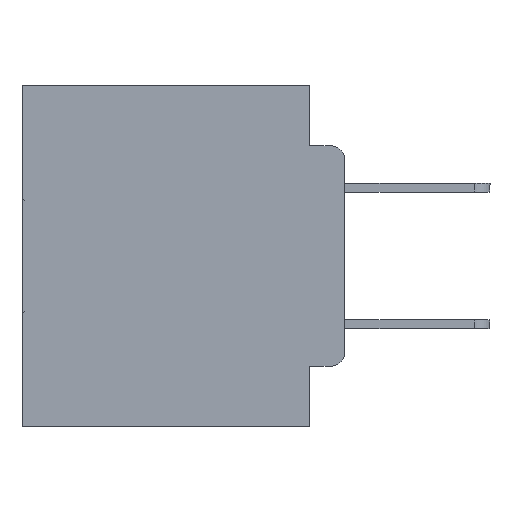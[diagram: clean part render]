
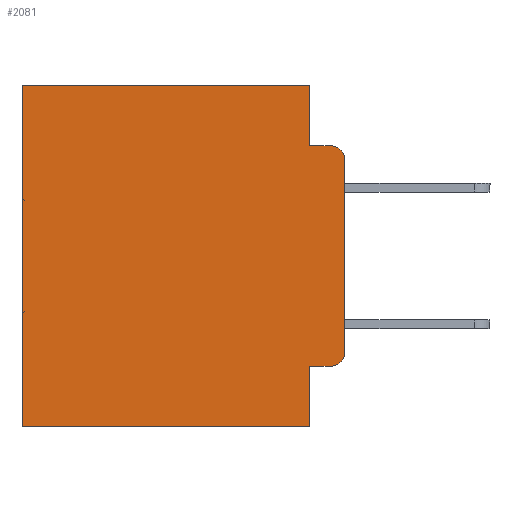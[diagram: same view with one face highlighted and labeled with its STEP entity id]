
A CAD part, left-side view. The second image highlights one B-rep face of the part: STEP entity #2081.
In plain terms, the highlighted planar face has unit normal (-1, 0, 0).
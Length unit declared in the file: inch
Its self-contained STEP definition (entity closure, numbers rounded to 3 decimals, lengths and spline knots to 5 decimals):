
#82 = CARTESIAN_POINT ( 'NONE',  ( 0.298, 0.473, -0.5 ) ) ;
#234 = CARTESIAN_POINT ( 'NONE',  ( 0.298, 0.473, 0. ) ) ;
#344 = ORIENTED_EDGE ( 'NONE', *, *, #11856, .F. ) ;
#406 = VECTOR ( 'NONE', #6582, 39.37008 ) ;
#436 = LINE ( 'NONE', #24185, #19536 ) ;
#500 = VECTOR ( 'NONE', #5711, 39.37008 ) ;
#1049 = ORIENTED_EDGE ( 'NONE', *, *, #2192, .F. ) ;
#1088 = LINE ( 'NONE', #22377, #31598 ) ;
#1251 = DIRECTION ( 'NONE',  ( -1., 0., 0. ) ) ;
#1315 = LINE ( 'NONE', #20563, #500 ) ;
#1453 = EDGE_LOOP ( 'NONE', ( #344, #12089, #8398, #3783, #7740, #3040, #1049, #2171, #7056, #9646 ) ) ;
#1758 = EDGE_CURVE ( 'NONE', #31457, #2071, #436, .T. ) ;
#2012 = CARTESIAN_POINT ( 'NONE',  ( 0.298, 0.051, -0.5 ) ) ;
#2071 = VERTEX_POINT ( 'NONE', #4036 ) ;
#2081 = ADVANCED_FACE ( 'NONE', ( #30602 ), #30395, .F. ) ;
#2091 = DIRECTION ( 'NONE',  ( 0., -1., 0. ) ) ;
#2171 = ORIENTED_EDGE ( 'NONE', *, *, #20713, .F. ) ;
#2192 = EDGE_CURVE ( 'NONE', #28449, #8129, #26793, .T. ) ;
#2549 = CARTESIAN_POINT ( 'NONE',  ( 0.298, 0.051, -0.4115 ) ) ;
#2561 = CARTESIAN_POINT ( 'NONE',  ( 0.298, 0.051, 0. ) ) ;
#3040 = ORIENTED_EDGE ( 'NONE', *, *, #22358, .T. ) ;
#3138 = CARTESIAN_POINT ( 'NONE',  ( 0.298, 0., -0.1085 ) ) ;
#3783 = ORIENTED_EDGE ( 'NONE', *, *, #27270, .F. ) ;
#4036 = CARTESIAN_POINT ( 'NONE',  ( 0.298, 0.02, -0.0885 ) ) ;
#4209 = VERTEX_POINT ( 'NONE', #234 ) ;
#5115 = DIRECTION ( 'NONE',  ( 0., 0., -1. ) ) ;
#5131 = EDGE_CURVE ( 'NONE', #28104, #2071, #10438, .T. ) ;
#5205 = VERTEX_POINT ( 'NONE', #13309 ) ;
#5264 = CARTESIAN_POINT ( 'NONE',  ( 0.298, 0.473, 0. ) ) ;
#5711 = DIRECTION ( 'NONE',  ( 0., 1., 0. ) ) ;
#6582 = DIRECTION ( 'NONE',  ( 0., 1., 0. ) ) ;
#7056 = ORIENTED_EDGE ( 'NONE', *, *, #12464, .T. ) ;
#7740 = ORIENTED_EDGE ( 'NONE', *, *, #15792, .T. ) ;
#8129 = VERTEX_POINT ( 'NONE', #82 ) ;
#8398 = ORIENTED_EDGE ( 'NONE', *, *, #1758, .F. ) ;
#8658 = LINE ( 'NONE', #2549, #21014 ) ;
#9132 = EDGE_CURVE ( 'NONE', #31596, #11874, #24035, .T. ) ;
#9646 = ORIENTED_EDGE ( 'NONE', *, *, #9132, .T. ) ;
#10153 = DIRECTION ( 'NONE',  ( 0., 0., -1. ) ) ;
#10220 = CARTESIAN_POINT ( 'NONE',  ( 0.298, 0.02, -0.1085 ) ) ;
#10438 = CIRCLE ( 'NONE', #16133, 0.02 ) ;
#11856 = EDGE_CURVE ( 'NONE', #28104, #11874, #26385, .T. ) ;
#11874 = VERTEX_POINT ( 'NONE', #29782 ) ;
#12089 = ORIENTED_EDGE ( 'NONE', *, *, #5131, .T. ) ;
#12464 = EDGE_CURVE ( 'NONE', #5205, #31596, #8658, .T. ) ;
#12546 = CARTESIAN_POINT ( 'NONE',  ( 0.298, 0.02, -0.4115 ) ) ;
#13309 = CARTESIAN_POINT ( 'NONE',  ( 0.298, 0.051, -0.4115 ) ) ;
#14399 = CARTESIAN_POINT ( 'NONE',  ( 0.298, 0.02, -0.3915 ) ) ;
#14442 = LINE ( 'NONE', #5264, #21781 ) ;
#15792 = EDGE_CURVE ( 'NONE', #24502, #4209, #1315, .T. ) ;
#16133 = AXIS2_PLACEMENT_3D ( 'NONE', #10220, #1251, #10153 ) ;
#16844 = DIRECTION ( 'NONE',  ( 0., 0., -1. ) ) ;
#17233 = VECTOR ( 'NONE', #27936, 39.37008 ) ;
#17857 = AXIS2_PLACEMENT_3D ( 'NONE', #14399, #31499, #16844 ) ;
#17874 = CARTESIAN_POINT ( 'NONE',  ( 0.298, 0., -0.5 ) ) ;
#18517 = AXIS2_PLACEMENT_3D ( 'NONE', #22506, #21951, #21909 ) ;
#19536 = VECTOR ( 'NONE', #2091, 39.37008 ) ;
#19902 = DIRECTION ( 'NONE',  ( 0., 0., -1. ) ) ;
#19928 = DIRECTION ( 'NONE',  ( 0., -1., 0. ) ) ;
#20445 = CARTESIAN_POINT ( 'NONE',  ( 0.298, 0.051, 0. ) ) ;
#20563 = CARTESIAN_POINT ( 'NONE',  ( 0.298, 0., 0. ) ) ;
#20683 = VECTOR ( 'NONE', #5115, 39.37008 ) ;
#20713 = EDGE_CURVE ( 'NONE', #5205, #28449, #23780, .T. ) ;
#21014 = VECTOR ( 'NONE', #19928, 39.37008 ) ;
#21781 = VECTOR ( 'NONE', #22585, 39.37008 ) ;
#21909 = DIRECTION ( 'NONE',  ( 0., 0., -1. ) ) ;
#21951 = DIRECTION ( 'NONE',  ( 1., 0., 0. ) ) ;
#22358 = EDGE_CURVE ( 'NONE', #4209, #8129, #14442, .T. ) ;
#22377 = CARTESIAN_POINT ( 'NONE',  ( 0.298, 0.051, 0. ) ) ;
#22444 = CARTESIAN_POINT ( 'NONE',  ( 0.298, 0., 0. ) ) ;
#22506 = CARTESIAN_POINT ( 'NONE',  ( 0.298, 0., 0. ) ) ;
#22585 = DIRECTION ( 'NONE',  ( 0., 0., -1. ) ) ;
#23780 = LINE ( 'NONE', #20445, #17233 ) ;
#24035 = CIRCLE ( 'NONE', #17857, 0.02 ) ;
#24185 = CARTESIAN_POINT ( 'NONE',  ( 0.298, 0.051, -0.0885 ) ) ;
#24247 = CARTESIAN_POINT ( 'NONE',  ( 0.298, 0.051, -0.0885 ) ) ;
#24502 = VERTEX_POINT ( 'NONE', #2561 ) ;
#26385 = LINE ( 'NONE', #22444, #20683 ) ;
#26793 = LINE ( 'NONE', #17874, #406 ) ;
#27270 = EDGE_CURVE ( 'NONE', #24502, #31457, #1088, .T. ) ;
#27936 = DIRECTION ( 'NONE',  ( 0., 0., -1. ) ) ;
#28104 = VERTEX_POINT ( 'NONE', #3138 ) ;
#28449 = VERTEX_POINT ( 'NONE', #2012 ) ;
#29782 = CARTESIAN_POINT ( 'NONE',  ( 0.298, 0., -0.3915 ) ) ;
#30395 = PLANE ( 'NONE',  #18517 ) ;
#30602 = FACE_OUTER_BOUND ( 'NONE', #1453, .T. ) ;
#31457 = VERTEX_POINT ( 'NONE', #24247 ) ;
#31499 = DIRECTION ( 'NONE',  ( -1., 0., 0. ) ) ;
#31596 = VERTEX_POINT ( 'NONE', #12546 ) ;
#31598 = VECTOR ( 'NONE', #19902, 39.37008 ) ;
